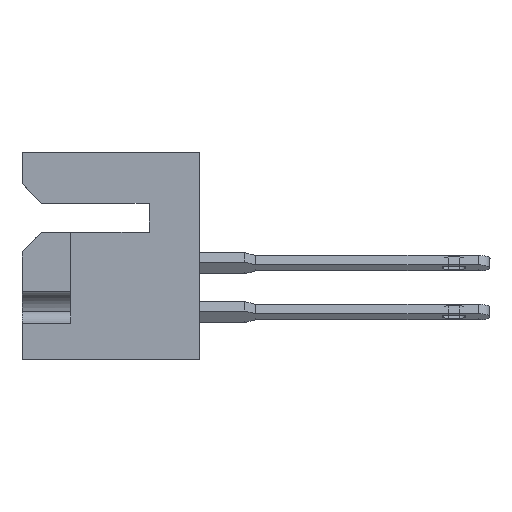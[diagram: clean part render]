
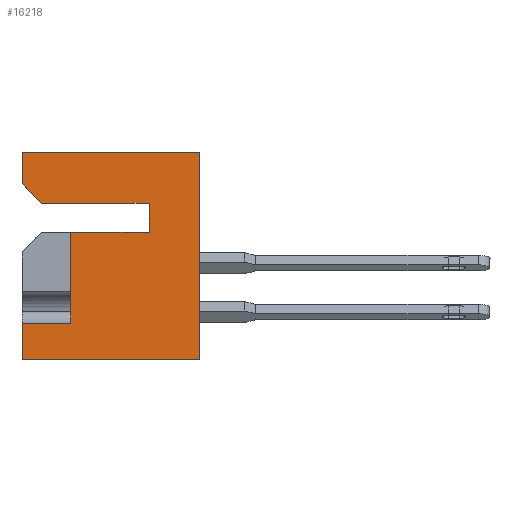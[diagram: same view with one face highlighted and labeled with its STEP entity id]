
A CAD part, left-side view. The second image highlights one B-rep face of the part: STEP entity #16218.
In plain terms, the highlighted planar face has unit normal (-1, 0, 0).
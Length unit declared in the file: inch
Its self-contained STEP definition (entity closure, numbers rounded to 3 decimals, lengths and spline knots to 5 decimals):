
#24 = EDGE_CURVE ( 'NONE', #14165, #9561, #12465, .T. ) ;
#125 = ORIENTED_EDGE ( 'NONE', *, *, #13801, .T. ) ;
#356 = VECTOR ( 'NONE', #26892, 39.37008 ) ;
#852 = DIRECTION ( 'NONE',  ( 0., -1., 0. ) ) ;
#916 = DIRECTION ( 'NONE',  ( 0., 0., 1. ) ) ;
#949 = LINE ( 'NONE', #7535, #5816 ) ;
#1123 = VECTOR ( 'NONE', #27786, 39.37008 ) ;
#1197 = EDGE_CURVE ( 'NONE', #16281, #23622, #1876, .T. ) ;
#1876 = LINE ( 'NONE', #11092, #1123 ) ;
#2395 = ORIENTED_EDGE ( 'NONE', *, *, #20509, .F. ) ;
#2492 = EDGE_CURVE ( 'NONE', #14876, #11720, #11846, .T. ) ;
#2604 = LINE ( 'NONE', #26039, #20569 ) ;
#2858 = VECTOR ( 'NONE', #10031, 39.37008 ) ;
#2885 = CARTESIAN_POINT ( 'NONE',  ( 0., 0.453, 0. ) ) ;
#2940 = CARTESIAN_POINT ( 'NONE',  ( 0., 0.453, 0. ) ) ;
#3090 = VECTOR ( 'NONE', #24661, 39.37008 ) ;
#3100 = ORIENTED_EDGE ( 'NONE', *, *, #24, .F. ) ;
#4504 = CARTESIAN_POINT ( 'NONE',  ( 0., 0.453, 0. ) ) ;
#4958 = DIRECTION ( 'NONE',  ( 0., 1., 0. ) ) ;
#5208 = ORIENTED_EDGE ( 'NONE', *, *, #1197, .T. ) ;
#5312 = ORIENTED_EDGE ( 'NONE', *, *, #26961, .F. ) ;
#5377 = VERTEX_POINT ( 'NONE', #12306 ) ;
#5816 = VECTOR ( 'NONE', #19847, 39.37008 ) ;
#5944 = CARTESIAN_POINT ( 'NONE',  ( 0., 0.453, 0. ) ) ;
#5949 = CARTESIAN_POINT ( 'NONE',  ( 0., 0.328, -0.437 ) ) ;
#6599 = PLANE ( 'NONE',  #11927 ) ;
#7535 = CARTESIAN_POINT ( 'NONE',  ( 0., 0.453, 0. ) ) ;
#8334 = LINE ( 'NONE', #2885, #11687 ) ;
#9024 = DIRECTION ( 'NONE',  ( 0., 0., -1. ) ) ;
#9561 = VERTEX_POINT ( 'NONE', #10959 ) ;
#10031 = DIRECTION ( 'NONE',  ( 0., 0., 1. ) ) ;
#10206 = CARTESIAN_POINT ( 'NONE',  ( 0., 0.128, -0.131 ) ) ;
#10443 = CARTESIAN_POINT ( 'NONE',  ( 0., 0.328, -0.205 ) ) ;
#10959 = CARTESIAN_POINT ( 'NONE',  ( 0., 0., 0. ) ) ;
#11092 = CARTESIAN_POINT ( 'NONE',  ( 0., 0.403, -0.131 ) ) ;
#11491 = EDGE_CURVE ( 'NONE', #28510, #12880, #26499, .T. ) ;
#11687 = VECTOR ( 'NONE', #29006, 39.37008 ) ;
#11720 = VERTEX_POINT ( 'NONE', #17383 ) ;
#11749 = DIRECTION ( 'NONE',  ( 0., 1., 0. ) ) ;
#11846 = LINE ( 'NONE', #24672, #27176 ) ;
#11927 = AXIS2_PLACEMENT_3D ( 'NONE', #4504, #13790, #9024 ) ;
#12306 = CARTESIAN_POINT ( 'NONE',  ( 0., 0.128, -0.131 ) ) ;
#12465 = LINE ( 'NONE', #2940, #3090 ) ;
#12704 = EDGE_CURVE ( 'NONE', #11720, #9561, #26781, .T. ) ;
#12880 = VERTEX_POINT ( 'NONE', #10443 ) ;
#13790 = DIRECTION ( 'NONE',  ( 1., 0., 0. ) ) ;
#13801 = EDGE_CURVE ( 'NONE', #28160, #29212, #2604, .T. ) ;
#14165 = VERTEX_POINT ( 'NONE', #5944 ) ;
#14445 = CARTESIAN_POINT ( 'NONE',  ( 0., 0.128, -0.205 ) ) ;
#14876 = VERTEX_POINT ( 'NONE', #15607 ) ;
#15292 = LINE ( 'NONE', #10206, #356 ) ;
#15607 = CARTESIAN_POINT ( 'NONE',  ( 0., 0.453, -0.531 ) ) ;
#15776 = CARTESIAN_POINT ( 'NONE',  ( 0., 0.403, -0.131 ) ) ;
#16108 = ORIENTED_EDGE ( 'NONE', *, *, #2492, .T. ) ;
#16218 = ADVANCED_FACE ( 'NONE', ( #30149 ), #6599, .F. ) ;
#16281 = VERTEX_POINT ( 'NONE', #21102 ) ;
#16373 = ORIENTED_EDGE ( 'NONE', *, *, #24511, .F. ) ;
#17018 = ORIENTED_EDGE ( 'NONE', *, *, #11491, .T. ) ;
#17069 = EDGE_CURVE ( 'NONE', #14876, #29212, #949, .T. ) ;
#17383 = CARTESIAN_POINT ( 'NONE',  ( 0., 0., -0.531 ) ) ;
#17484 = LINE ( 'NONE', #20381, #27945 ) ;
#18913 = CARTESIAN_POINT ( 'NONE',  ( 0., 0., 0. ) ) ;
#19745 = CARTESIAN_POINT ( 'NONE',  ( 0., 0.328, -0.205 ) ) ;
#19750 = CARTESIAN_POINT ( 'NONE',  ( 0., 0.453, -0.437 ) ) ;
#19847 = DIRECTION ( 'NONE',  ( 0., 0., 1. ) ) ;
#19994 = CARTESIAN_POINT ( 'NONE',  ( 0., 0.128, -0.205 ) ) ;
#20381 = CARTESIAN_POINT ( 'NONE',  ( 0., 0.128, -0.131 ) ) ;
#20509 = EDGE_CURVE ( 'NONE', #5377, #23622, #15292, .T. ) ;
#20569 = VECTOR ( 'NONE', #11749, 39.37008 ) ;
#21102 = CARTESIAN_POINT ( 'NONE',  ( 0., 0.453, -0.081 ) ) ;
#21974 = ORIENTED_EDGE ( 'NONE', *, *, #12704, .T. ) ;
#23622 = VERTEX_POINT ( 'NONE', #15776 ) ;
#23905 = EDGE_CURVE ( 'NONE', #28160, #12880, #30021, .T. ) ;
#24511 = EDGE_CURVE ( 'NONE', #16281, #14165, #8334, .T. ) ;
#24661 = DIRECTION ( 'NONE',  ( 0., -1., 0. ) ) ;
#24672 = CARTESIAN_POINT ( 'NONE',  ( 0., 0.453, -0.531 ) ) ;
#26039 = CARTESIAN_POINT ( 'NONE',  ( 0., 0.328, -0.437 ) ) ;
#26499 = LINE ( 'NONE', #14445, #29109 ) ;
#26781 = LINE ( 'NONE', #18913, #2858 ) ;
#26892 = DIRECTION ( 'NONE',  ( 0., 1., 0. ) ) ;
#26961 = EDGE_CURVE ( 'NONE', #28510, #5377, #17484, .T. ) ;
#27073 = ORIENTED_EDGE ( 'NONE', *, *, #23905, .F. ) ;
#27176 = VECTOR ( 'NONE', #852, 39.37008 ) ;
#27638 = EDGE_LOOP ( 'NONE', ( #125, #29653, #16108, #21974, #3100, #16373, #5208, #2395, #5312, #17018, #27073 ) ) ;
#27695 = DIRECTION ( 'NONE',  ( 0., 0., 1. ) ) ;
#27786 = DIRECTION ( 'NONE',  ( 0., -0.707, -0.707 ) ) ;
#27945 = VECTOR ( 'NONE', #27695, 39.37008 ) ;
#28160 = VERTEX_POINT ( 'NONE', #5949 ) ;
#28510 = VERTEX_POINT ( 'NONE', #19994 ) ;
#28554 = VECTOR ( 'NONE', #916, 39.37008 ) ;
#29006 = DIRECTION ( 'NONE',  ( 0., 0., 1. ) ) ;
#29109 = VECTOR ( 'NONE', #4958, 39.37008 ) ;
#29212 = VERTEX_POINT ( 'NONE', #19750 ) ;
#29653 = ORIENTED_EDGE ( 'NONE', *, *, #17069, .F. ) ;
#30021 = LINE ( 'NONE', #19745, #28554 ) ;
#30149 = FACE_OUTER_BOUND ( 'NONE', #27638, .T. ) ;
